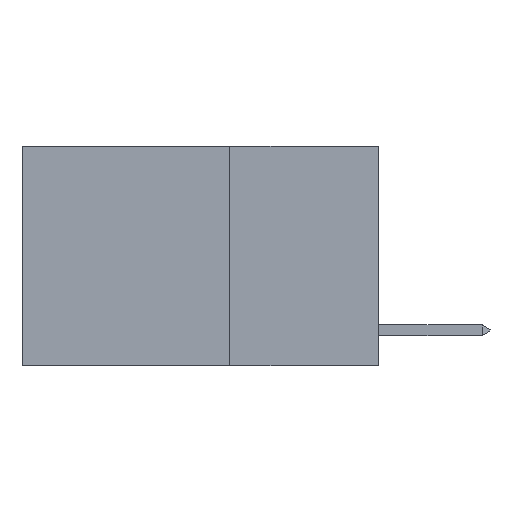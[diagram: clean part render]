
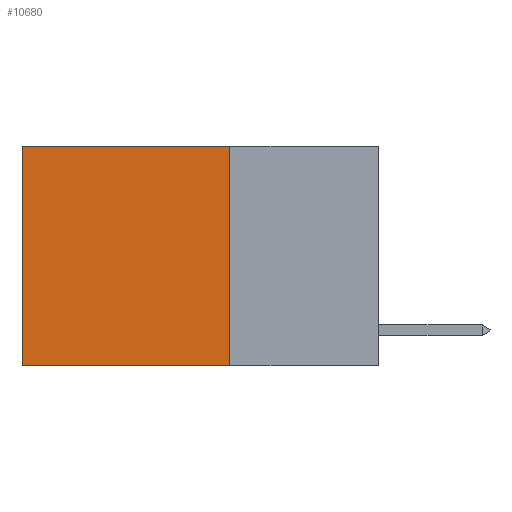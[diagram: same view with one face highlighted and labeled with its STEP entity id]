
A CAD part, left-side view. The second image highlights one B-rep face of the part: STEP entity #10680.
In plain terms, the highlighted planar face has unit normal (-1, 0, 0).
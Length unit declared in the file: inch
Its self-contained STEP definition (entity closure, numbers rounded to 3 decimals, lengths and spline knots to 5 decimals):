
#30 = ORIENTED_EDGE ( 'NONE', *, *, #1201, .T. ) ;
#163 = DIRECTION ( 'NONE',  ( 0., 1., 0. ) ) ;
#576 = DIRECTION ( 'NONE',  ( 0., 0., -1. ) ) ;
#1201 = EDGE_CURVE ( 'NONE', #18145, #14988, #2649, .T. ) ;
#1562 = CARTESIAN_POINT ( 'NONE',  ( 0.2625, 0.25, -0.37 ) ) ;
#1706 = VERTEX_POINT ( 'NONE', #1562 ) ;
#1975 = VERTEX_POINT ( 'NONE', #18778 ) ;
#2107 = DIRECTION ( 'NONE',  ( 1., 0., 0. ) ) ;
#2649 = LINE ( 'NONE', #14184, #16976 ) ;
#2767 = ORIENTED_EDGE ( 'NONE', *, *, #17461, .F. ) ;
#3648 = ORIENTED_EDGE ( 'NONE', *, *, #14219, .T. ) ;
#3658 = PLANE ( 'NONE',  #15761 ) ;
#4442 = EDGE_CURVE ( 'NONE', #1706, #1975, #5713, .T. ) ;
#4758 = VECTOR ( 'NONE', #11509, 39.37008 ) ;
#5261 = CARTESIAN_POINT ( 'NONE',  ( 0.2625, 0.25, 0. ) ) ;
#5713 = LINE ( 'NONE', #11028, #4758 ) ;
#7214 = CARTESIAN_POINT ( 'NONE',  ( 0.2625, 0.25, 0. ) ) ;
#7778 = LINE ( 'NONE', #5261, #13334 ) ;
#7809 = ORIENTED_EDGE ( 'NONE', *, *, #4442, .F. ) ;
#10680 = ADVANCED_FACE ( 'NONE', ( #13578 ), #3658, .F. ) ;
#11012 = LINE ( 'NONE', #19213, #17826 ) ;
#11028 = CARTESIAN_POINT ( 'NONE',  ( 0.2625, 0.25, -0.37 ) ) ;
#11509 = DIRECTION ( 'NONE',  ( 0., 1., 0. ) ) ;
#13334 = VECTOR ( 'NONE', #19100, 39.37008 ) ;
#13578 = FACE_OUTER_BOUND ( 'NONE', #19284, .T. ) ;
#14184 = CARTESIAN_POINT ( 'NONE',  ( 0.2625, 0.25, 0. ) ) ;
#14219 = EDGE_CURVE ( 'NONE', #14988, #1975, #11012, .T. ) ;
#14988 = VERTEX_POINT ( 'NONE', #16056 ) ;
#15761 = AXIS2_PLACEMENT_3D ( 'NONE', #16018, #2107, #19201 ) ;
#16018 = CARTESIAN_POINT ( 'NONE',  ( 0.2625, 0.25, 0. ) ) ;
#16056 = CARTESIAN_POINT ( 'NONE',  ( 0.2625, 0.6, 0. ) ) ;
#16976 = VECTOR ( 'NONE', #163, 39.37008 ) ;
#17461 = EDGE_CURVE ( 'NONE', #18145, #1706, #7778, .T. ) ;
#17826 = VECTOR ( 'NONE', #576, 39.37008 ) ;
#18145 = VERTEX_POINT ( 'NONE', #7214 ) ;
#18778 = CARTESIAN_POINT ( 'NONE',  ( 0.2625, 0.6, -0.37 ) ) ;
#19100 = DIRECTION ( 'NONE',  ( 0., 0., -1. ) ) ;
#19201 = DIRECTION ( 'NONE',  ( 0., 0., -1. ) ) ;
#19213 = CARTESIAN_POINT ( 'NONE',  ( 0.2625, 0.6, 0. ) ) ;
#19284 = EDGE_LOOP ( 'NONE', ( #3648, #7809, #2767, #30 ) ) ;
